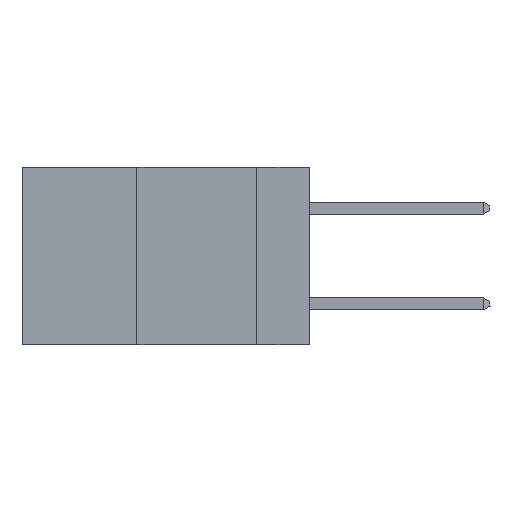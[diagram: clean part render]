
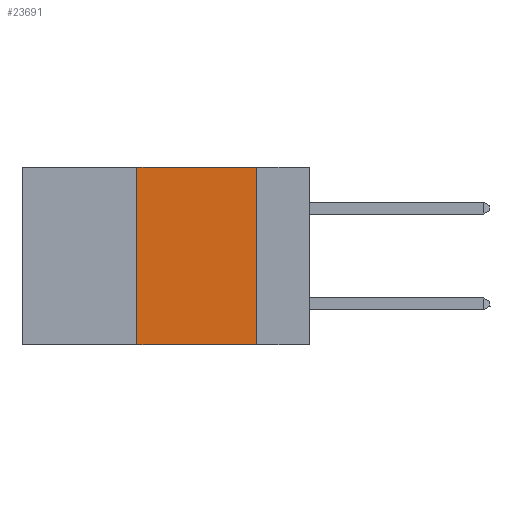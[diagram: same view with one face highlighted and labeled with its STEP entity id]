
A CAD part, left-side view. The second image highlights one B-rep face of the part: STEP entity #23691.
In plain terms, the highlighted planar face has unit normal (-1, 0, 0).
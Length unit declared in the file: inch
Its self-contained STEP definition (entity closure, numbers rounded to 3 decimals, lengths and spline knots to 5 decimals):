
#658 = DIRECTION ( 'NONE',  ( 0., 0., -1. ) ) ;
#1506 = DIRECTION ( 'NONE',  ( 0., -1., 0. ) ) ;
#1771 = VECTOR ( 'NONE', #658, 39.37008 ) ;
#3082 = DIRECTION ( 'NONE',  ( 0., 0., 1. ) ) ;
#5987 = CARTESIAN_POINT ( 'NONE',  ( 0., 0.6, 0. ) ) ;
#6031 = CARTESIAN_POINT ( 'NONE',  ( 0., 0.36, -0.37 ) ) ;
#6063 = LINE ( 'NONE', #6953, #23730 ) ;
#6937 = ORIENTED_EDGE ( 'NONE', *, *, #20129, .T. ) ;
#6953 = CARTESIAN_POINT ( 'NONE',  ( 0., 0.36, 0. ) ) ;
#7353 = FACE_OUTER_BOUND ( 'NONE', #14696, .T. ) ;
#7486 = CARTESIAN_POINT ( 'NONE',  ( 0., 0.11, -0.37 ) ) ;
#7790 = DIRECTION ( 'NONE',  ( 1., 0., 0. ) ) ;
#9000 = EDGE_CURVE ( 'NONE', #25809, #20738, #25241, .T. ) ;
#9133 = CARTESIAN_POINT ( 'NONE',  ( 0., 0.36, 0. ) ) ;
#9459 = LINE ( 'NONE', #21102, #1771 ) ;
#11503 = AXIS2_PLACEMENT_3D ( 'NONE', #5987, #7790, #22135 ) ;
#11861 = CARTESIAN_POINT ( 'NONE',  ( 0., 0.11, 0. ) ) ;
#12069 = CARTESIAN_POINT ( 'NONE',  ( 0., 0.6, 0. ) ) ;
#12980 = LINE ( 'NONE', #18427, #19123 ) ;
#13768 = ORIENTED_EDGE ( 'NONE', *, *, #16048, .F. ) ;
#14011 = VECTOR ( 'NONE', #1506, 39.37008 ) ;
#14696 = EDGE_LOOP ( 'NONE', ( #13768, #17729, #21889, #6937 ) ) ;
#16048 = EDGE_CURVE ( 'NONE', #20738, #22433, #9459, .T. ) ;
#16202 = DIRECTION ( 'NONE',  ( 0., -1., 0. ) ) ;
#17729 = ORIENTED_EDGE ( 'NONE', *, *, #9000, .F. ) ;
#18427 = CARTESIAN_POINT ( 'NONE',  ( 0., 0.6, -0.37 ) ) ;
#19123 = VECTOR ( 'NONE', #16202, 39.37008 ) ;
#20129 = EDGE_CURVE ( 'NONE', #23319, #22433, #12980, .T. ) ;
#20334 = PLANE ( 'NONE',  #11503 ) ;
#20738 = VERTEX_POINT ( 'NONE', #11861 ) ;
#21102 = CARTESIAN_POINT ( 'NONE',  ( 0., 0.11, 0. ) ) ;
#21889 = ORIENTED_EDGE ( 'NONE', *, *, #24146, .F. ) ;
#22135 = DIRECTION ( 'NONE',  ( 0., 0., -1. ) ) ;
#22433 = VERTEX_POINT ( 'NONE', #7486 ) ;
#23319 = VERTEX_POINT ( 'NONE', #6031 ) ;
#23691 = ADVANCED_FACE ( 'NONE', ( #7353 ), #20334, .F. ) ;
#23730 = VECTOR ( 'NONE', #3082, 39.37008 ) ;
#24146 = EDGE_CURVE ( 'NONE', #23319, #25809, #6063, .T. ) ;
#25241 = LINE ( 'NONE', #12069, #14011 ) ;
#25809 = VERTEX_POINT ( 'NONE', #9133 ) ;
